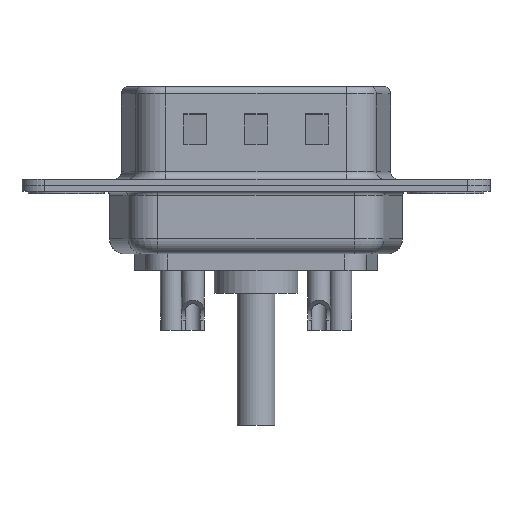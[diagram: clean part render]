
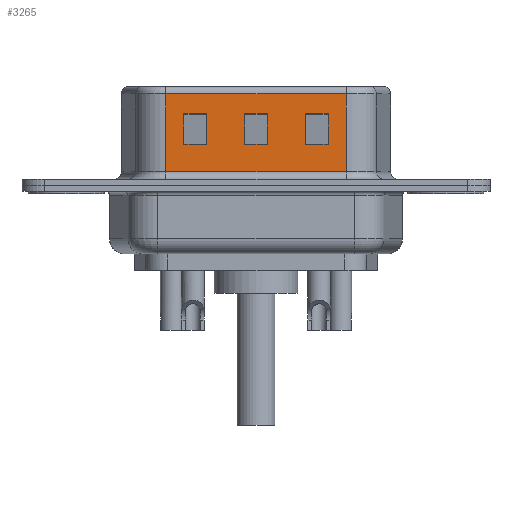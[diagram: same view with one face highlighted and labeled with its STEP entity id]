
A CAD part, front view. The second image highlights one B-rep face of the part: STEP entity #3265.
In plain terms, the highlighted planar face has unit normal (0, -1, 0).
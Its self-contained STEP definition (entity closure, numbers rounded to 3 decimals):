
#18 = DIRECTION ( 'NONE',  ( 0., 0., 1. ) ) ;
#61 = VERTEX_POINT ( 'NONE', #11736 ) ;
#168 = VERTEX_POINT ( 'NONE', #2552 ) ;
#386 = ORIENTED_EDGE ( 'NONE', *, *, #7073, .T. ) ;
#397 = LINE ( 'NONE', #9639, #2715 ) ;
#605 = LINE ( 'NONE', #3414, #6446 ) ;
#712 = VERTEX_POINT ( 'NONE', #11421 ) ;
#837 = VERTEX_POINT ( 'NONE', #10537 ) ;
#952 = LINE ( 'NONE', #10791, #11212 ) ;
#1039 = LINE ( 'NONE', #3487, #5951 ) ;
#1076 = CARTESIAN_POINT ( 'NONE',  ( 11.75, -4.58, 4.705 ) ) ;
#1391 = EDGE_LOOP ( 'NONE', ( #1895, #8017, #10258, #9702 ) ) ;
#1490 = AXIS2_PLACEMENT_3D ( 'NONE', #3730, #3997, #9597 ) ;
#1608 = VERTEX_POINT ( 'NONE', #1076 ) ;
#1632 = CARTESIAN_POINT ( 'NONE',  ( 13.25, -4.58, 6.52 ) ) ;
#1673 = VECTOR ( 'NONE', #4930, 1000. ) ;
#1709 = DIRECTION ( 'NONE',  ( -1., 0., 0. ) ) ;
#1850 = EDGE_CURVE ( 'NONE', #2046, #837, #9716, .T. ) ;
#1895 = ORIENTED_EDGE ( 'NONE', *, *, #4491, .T. ) ;
#1965 = LINE ( 'NONE', #3463, #11886 ) ;
#1983 = DIRECTION ( 'NONE',  ( 0., 0., -1. ) ) ;
#2046 = VERTEX_POINT ( 'NONE', #11218 ) ;
#2050 = EDGE_CURVE ( 'NONE', #8856, #10855, #2445, .T. ) ;
#2275 = ORIENTED_EDGE ( 'NONE', *, *, #7508, .T. ) ;
#2445 = LINE ( 'NONE', #4605, #5055 ) ;
#2552 = CARTESIAN_POINT ( 'NONE',  ( 9.25, -4.58, 2.705 ) ) ;
#2578 = VECTOR ( 'NONE', #11826, 1000. ) ;
#2594 = VECTOR ( 'NONE', #10513, 1000. ) ;
#2715 = VECTOR ( 'NONE', #6068, 1000. ) ;
#2716 = EDGE_CURVE ( 'NONE', #7770, #6452, #11082, .T. ) ;
#2879 = EDGE_CURVE ( 'NONE', #7009, #7172, #7134, .T. ) ;
#2880 = LINE ( 'NONE', #11772, #2578 ) ;
#3082 = VECTOR ( 'NONE', #8521, 1000. ) ;
#3140 = ORIENTED_EDGE ( 'NONE', *, *, #9634, .T. ) ;
#3172 = FACE_OUTER_BOUND ( 'NONE', #12388, .T. ) ;
#3265 = ADVANCED_FACE ( 'NONE', ( #5450, #10505, #8037, #3172 ), #9779, .F. ) ;
#3306 = VECTOR ( 'NONE', #11325, 1000. ) ;
#3388 = DIRECTION ( 'NONE',  ( 0., 0., 1. ) ) ;
#3414 = CARTESIAN_POINT ( 'NONE',  ( 18.45, -4.58, 2.705 ) ) ;
#3457 = ORIENTED_EDGE ( 'NONE', *, *, #7477, .T. ) ;
#3463 = CARTESIAN_POINT ( 'NONE',  ( 18.45, -4.58, 4.705 ) ) ;
#3487 = CARTESIAN_POINT ( 'NONE',  ( 11.75, -4.58, 6.52 ) ) ;
#3490 = VECTOR ( 'NONE', #5237, 1000. ) ;
#3730 = CARTESIAN_POINT ( 'NONE',  ( 18.45, -4.58, 6.52 ) ) ;
#3787 = VECTOR ( 'NONE', #1983, 1000. ) ;
#3834 = CARTESIAN_POINT ( 'NONE',  ( 22.45, -4.58, 2.705 ) ) ;
#3961 = EDGE_LOOP ( 'NONE', ( #7151, #9536, #7142, #4292 ) ) ;
#3997 = DIRECTION ( 'NONE',  ( 0., 1., 0. ) ) ;
#4064 = EDGE_CURVE ( 'NONE', #168, #8540, #952, .T. ) ;
#4292 = ORIENTED_EDGE ( 'NONE', *, *, #2879, .T. ) ;
#4322 = LINE ( 'NONE', #1632, #1673 ) ;
#4477 = CARTESIAN_POINT ( 'NONE',  ( 9.25, -4.58, 4.705 ) ) ;
#4491 = EDGE_CURVE ( 'NONE', #10855, #168, #11504, .T. ) ;
#4565 = VECTOR ( 'NONE', #10306, 1000. ) ;
#4605 = CARTESIAN_POINT ( 'NONE',  ( 14.45, -4.58, 4.705 ) ) ;
#4617 = LINE ( 'NONE', #4693, #6893 ) ;
#4693 = CARTESIAN_POINT ( 'NONE',  ( 7.75, -4.58, 6.52 ) ) ;
#4748 = CARTESIAN_POINT ( 'NONE',  ( 18.45, -4.58, 0.9 ) ) ;
#4930 = DIRECTION ( 'NONE',  ( 0., 0., -1. ) ) ;
#4968 = CARTESIAN_POINT ( 'NONE',  ( 6.55, -4.58, 6.52 ) ) ;
#5055 = VECTOR ( 'NONE', #11208, 1000. ) ;
#5101 = VERTEX_POINT ( 'NONE', #4748 ) ;
#5237 = DIRECTION ( 'NONE',  ( -1., 0., 0. ) ) ;
#5450 = FACE_BOUND ( 'NONE', #1391, .T. ) ;
#5469 = CARTESIAN_POINT ( 'NONE',  ( 17.25, -4.58, 2.705 ) ) ;
#5653 = VECTOR ( 'NONE', #9371, 1000. ) ;
#5749 = CARTESIAN_POINT ( 'NONE',  ( 7.75, -4.58, 2.705 ) ) ;
#5750 = CARTESIAN_POINT ( 'NONE',  ( 22.45, -4.58, 4.705 ) ) ;
#5938 = LINE ( 'NONE', #9435, #5653 ) ;
#5951 = VECTOR ( 'NONE', #3388, 1000. ) ;
#6068 = DIRECTION ( 'NONE',  ( -1., 0., 0. ) ) ;
#6248 = EDGE_CURVE ( 'NONE', #9591, #10288, #605, .T. ) ;
#6374 = LINE ( 'NONE', #12516, #3787 ) ;
#6446 = VECTOR ( 'NONE', #10640, 1000. ) ;
#6452 = VERTEX_POINT ( 'NONE', #7042 ) ;
#6893 = VECTOR ( 'NONE', #18, 1000. ) ;
#7009 = VERTEX_POINT ( 'NONE', #7950 ) ;
#7042 = CARTESIAN_POINT ( 'NONE',  ( 15.75, -4.58, 2.705 ) ) ;
#7073 = EDGE_CURVE ( 'NONE', #837, #5101, #10148, .T. ) ;
#7134 = LINE ( 'NONE', #5750, #4565 ) ;
#7142 = ORIENTED_EDGE ( 'NONE', *, *, #7731, .T. ) ;
#7151 = ORIENTED_EDGE ( 'NONE', *, *, #11476, .T. ) ;
#7172 = VERTEX_POINT ( 'NONE', #8535 ) ;
#7447 = EDGE_CURVE ( 'NONE', #8540, #8856, #4617, .T. ) ;
#7456 = ORIENTED_EDGE ( 'NONE', *, *, #6248, .T. ) ;
#7477 = EDGE_CURVE ( 'NONE', #61, #9591, #4322, .T. ) ;
#7482 = ORIENTED_EDGE ( 'NONE', *, *, #1850, .T. ) ;
#7508 = EDGE_CURVE ( 'NONE', #10288, #1608, #1039, .T. ) ;
#7731 = EDGE_CURVE ( 'NONE', #6452, #7009, #2880, .T. ) ;
#7770 = VERTEX_POINT ( 'NONE', #5469 ) ;
#7950 = CARTESIAN_POINT ( 'NONE',  ( 15.75, -4.58, 4.705 ) ) ;
#8017 = ORIENTED_EDGE ( 'NONE', *, *, #4064, .T. ) ;
#8037 = FACE_BOUND ( 'NONE', #8731, .T. ) ;
#8415 = DIRECTION ( 'NONE',  ( 1., 0., 0. ) ) ;
#8447 = EDGE_CURVE ( 'NONE', #712, #2046, #397, .T. ) ;
#8521 = DIRECTION ( 'NONE',  ( 1., 0., 0. ) ) ;
#8535 = CARTESIAN_POINT ( 'NONE',  ( 17.25, -4.58, 4.705 ) ) ;
#8540 = VERTEX_POINT ( 'NONE', #5749 ) ;
#8731 = EDGE_LOOP ( 'NONE', ( #3140, #3457, #7456, #2275 ) ) ;
#8856 = VERTEX_POINT ( 'NONE', #12064 ) ;
#9371 = DIRECTION ( 'NONE',  ( 0., 0., -1. ) ) ;
#9435 = CARTESIAN_POINT ( 'NONE',  ( 18.45, -4.58, 6.52 ) ) ;
#9536 = ORIENTED_EDGE ( 'NONE', *, *, #2716, .T. ) ;
#9591 = VERTEX_POINT ( 'NONE', #9707 ) ;
#9597 = DIRECTION ( 'NONE',  ( 0., 0., 1. ) ) ;
#9634 = EDGE_CURVE ( 'NONE', #1608, #61, #1965, .T. ) ;
#9639 = CARTESIAN_POINT ( 'NONE',  ( 18.45, -4.58, 6.02 ) ) ;
#9702 = ORIENTED_EDGE ( 'NONE', *, *, #2050, .T. ) ;
#9707 = CARTESIAN_POINT ( 'NONE',  ( 13.25, -4.58, 2.705 ) ) ;
#9716 = LINE ( 'NONE', #4968, #2594 ) ;
#9779 = PLANE ( 'NONE',  #1490 ) ;
#10148 = LINE ( 'NONE', #11134, #3082 ) ;
#10258 = ORIENTED_EDGE ( 'NONE', *, *, #7447, .T. ) ;
#10288 = VERTEX_POINT ( 'NONE', #10961 ) ;
#10306 = DIRECTION ( 'NONE',  ( 1., 0., 0. ) ) ;
#10458 = EDGE_CURVE ( 'NONE', #712, #5101, #5938, .T. ) ;
#10498 = CARTESIAN_POINT ( 'NONE',  ( 9.25, -4.58, 6.52 ) ) ;
#10505 = FACE_BOUND ( 'NONE', #3961, .T. ) ;
#10513 = DIRECTION ( 'NONE',  ( 0., 0., -1. ) ) ;
#10537 = CARTESIAN_POINT ( 'NONE',  ( 6.55, -4.58, 0.9 ) ) ;
#10640 = DIRECTION ( 'NONE',  ( -1., 0., 0. ) ) ;
#10700 = ORIENTED_EDGE ( 'NONE', *, *, #8447, .T. ) ;
#10791 = CARTESIAN_POINT ( 'NONE',  ( 14.45, -4.58, 2.705 ) ) ;
#10855 = VERTEX_POINT ( 'NONE', #4477 ) ;
#10961 = CARTESIAN_POINT ( 'NONE',  ( 11.75, -4.58, 2.705 ) ) ;
#11042 = ORIENTED_EDGE ( 'NONE', *, *, #10458, .F. ) ;
#11082 = LINE ( 'NONE', #3834, #3490 ) ;
#11134 = CARTESIAN_POINT ( 'NONE',  ( 18.45, -4.58, 0.9 ) ) ;
#11208 = DIRECTION ( 'NONE',  ( 1., 0., 0. ) ) ;
#11212 = VECTOR ( 'NONE', #1709, 1000. ) ;
#11218 = CARTESIAN_POINT ( 'NONE',  ( 6.55, -4.58, 6.02 ) ) ;
#11325 = DIRECTION ( 'NONE',  ( 0., 0., -1. ) ) ;
#11421 = CARTESIAN_POINT ( 'NONE',  ( 18.45, -4.58, 6.02 ) ) ;
#11476 = EDGE_CURVE ( 'NONE', #7172, #7770, #6374, .T. ) ;
#11504 = LINE ( 'NONE', #10498, #3306 ) ;
#11736 = CARTESIAN_POINT ( 'NONE',  ( 13.25, -4.58, 4.705 ) ) ;
#11772 = CARTESIAN_POINT ( 'NONE',  ( 15.75, -4.58, 6.52 ) ) ;
#11826 = DIRECTION ( 'NONE',  ( 0., 0., 1. ) ) ;
#11886 = VECTOR ( 'NONE', #8415, 1000. ) ;
#12064 = CARTESIAN_POINT ( 'NONE',  ( 7.75, -4.58, 4.705 ) ) ;
#12388 = EDGE_LOOP ( 'NONE', ( #11042, #10700, #7482, #386 ) ) ;
#12516 = CARTESIAN_POINT ( 'NONE',  ( 17.25, -4.58, 6.52 ) ) ;
